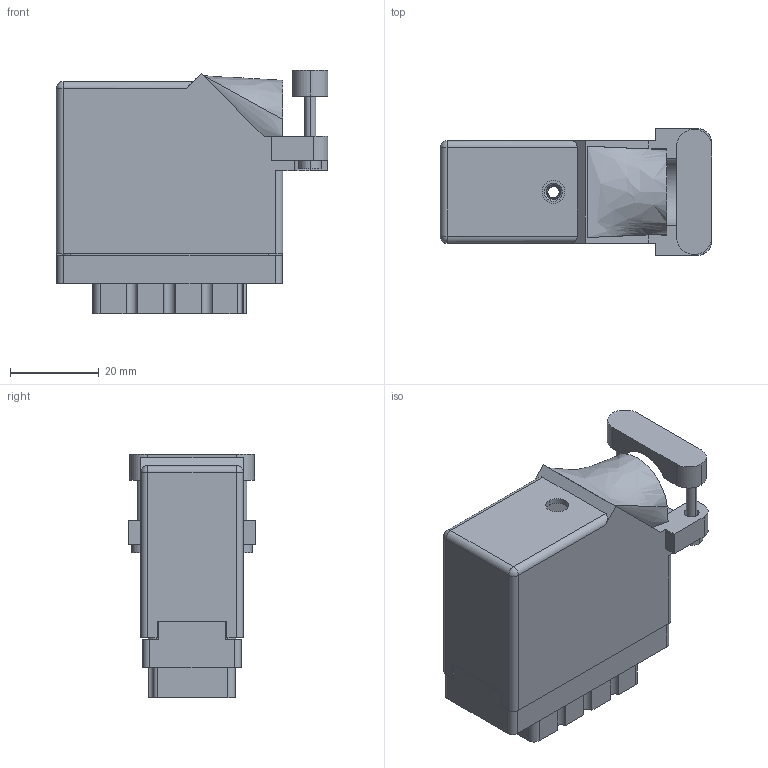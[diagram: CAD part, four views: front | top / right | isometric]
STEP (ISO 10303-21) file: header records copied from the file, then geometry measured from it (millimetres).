
FILE_DESCRIPTION (( 'STEP AP203' ), '1' );
FILE_NAME ('516-038-000-446.STEP', '2020-03-04T22:00:18', ( '' ), ( '' ), 'SwSTEP 2.0', 'SolidWorks 2016', '' );
FILE_SCHEMA (( 'CONFIG_CONTROL_DESIGN' ));
Length unit declared in the file: inch
Products named in the file (4): 516-038-000-446; 516-252-035-100_516-252-035-100; 516 Part Receptacle_038; 516-230-001_Plastic - 038 Side Entry - Large Clamp
Assembly tree (3 placements, depth 2):
  516-038-000-446
    516 Part Receptacle_038
    516-230-001_Plastic - 038 Side Entry - Large Clamp
    516-252-035-100_516-252-035-100
Bounding box: 61.21 x 28.57 x 54.91 mm (x, y, z)
Volume: 21764.1 mm3; surface area: 29210.7 mm2
Topology: 3 solids, 3 shells, 1051 faces, 3052 edges, 2028 vertices
Faces by surface type: plane 693, cylinder 335, cone 12, bspline 9, sphere 2
Entity records: 37668 total; most frequent: CARTESIAN_POINT 8674, ORIENTED_EDGE 6100, DIRECTION 5902, EDGE_CURVE 3050, VECTOR 2186, LINE 2186, VERTEX_POINT 2028, AXIS2_PLACEMENT_3D 1858
